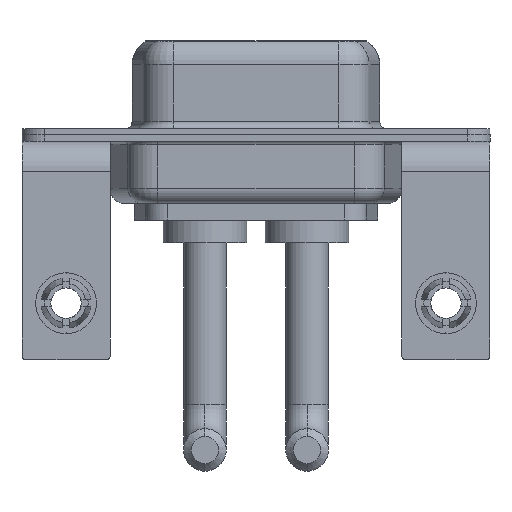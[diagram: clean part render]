
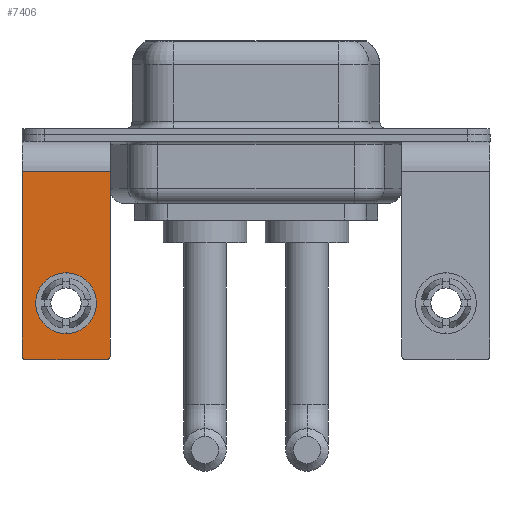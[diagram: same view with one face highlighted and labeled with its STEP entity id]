
A CAD part, front view. The second image highlights one B-rep face of the part: STEP entity #7406.
In plain terms, the highlighted planar face has unit normal (0, -1, 0).
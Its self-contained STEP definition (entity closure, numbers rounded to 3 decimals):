
#21 = VECTOR ( 'NONE', #13618, 1000. ) ;
#364 = CARTESIAN_POINT ( 'NONE',  ( 0., -6.25, -11.07 ) ) ;
#585 = DIRECTION ( 'NONE',  ( 0., -1., 0. ) ) ;
#714 = DIRECTION ( 'NONE',  ( -1., 0., 0. ) ) ;
#743 = ORIENTED_EDGE ( 'NONE', *, *, #3849, .F. ) ;
#789 = DIRECTION ( 'NONE',  ( 0., 1., 0. ) ) ;
#862 = CARTESIAN_POINT ( 'NONE',  ( 0., -6.25, -11.07 ) ) ;
#1031 = PLANE ( 'NONE',  #11080 ) ;
#1300 = EDGE_LOOP ( 'NONE', ( #14011, #5399, #4570, #6254, #743, #12865 ) ) ;
#1402 = VERTEX_POINT ( 'NONE', #13910 ) ;
#1481 = CARTESIAN_POINT ( 'NONE',  ( 0., -6.25, -13.07 ) ) ;
#1553 = CIRCLE ( 'NONE', #11958, 0.25 ) ;
#1920 = ORIENTED_EDGE ( 'NONE', *, *, #5499, .T. ) ;
#2193 = CARTESIAN_POINT ( 'NONE',  ( 2.9, -6.25, -14.55 ) ) ;
#2292 = VERTEX_POINT ( 'NONE', #8793 ) ;
#2634 = EDGE_CURVE ( 'NONE', #6233, #2292, #1553, .T. ) ;
#3094 = AXIS2_PLACEMENT_3D ( 'NONE', #862, #789, #9762 ) ;
#3145 = LINE ( 'NONE', #5505, #4520 ) ;
#3213 = CARTESIAN_POINT ( 'NONE',  ( 0., -6.25, -9.07 ) ) ;
#3627 = DIRECTION ( 'NONE',  ( 0., 0., -1. ) ) ;
#3849 = EDGE_CURVE ( 'NONE', #1402, #5705, #4943, .T. ) ;
#4283 = CARTESIAN_POINT ( 'NONE',  ( 2.65, -6.25, -14.8 ) ) ;
#4520 = VECTOR ( 'NONE', #714, 1000. ) ;
#4570 = ORIENTED_EDGE ( 'NONE', *, *, #10517, .F. ) ;
#4727 = DIRECTION ( 'NONE',  ( 0., 0., 1. ) ) ;
#4874 = LINE ( 'NONE', #5689, #21 ) ;
#4943 = LINE ( 'NONE', #10308, #11025 ) ;
#5083 = DIRECTION ( 'NONE',  ( 0., 0., 1. ) ) ;
#5118 = VERTEX_POINT ( 'NONE', #1481 ) ;
#5286 = VERTEX_POINT ( 'NONE', #4283 ) ;
#5399 = ORIENTED_EDGE ( 'NONE', *, *, #2634, .T. ) ;
#5499 = EDGE_CURVE ( 'NONE', #10412, #5118, #9878, .T. ) ;
#5505 = CARTESIAN_POINT ( 'NONE',  ( 2.9, -6.25, -2.4 ) ) ;
#5668 = DIRECTION ( 'NONE',  ( 0., 0., 1. ) ) ;
#5689 = CARTESIAN_POINT ( 'NONE',  ( -2.9, -6.25, -2.4 ) ) ;
#5705 = VERTEX_POINT ( 'NONE', #2193 ) ;
#5760 = EDGE_LOOP ( 'NONE', ( #13253, #1920 ) ) ;
#6233 = VERTEX_POINT ( 'NONE', #13499 ) ;
#6254 = ORIENTED_EDGE ( 'NONE', *, *, #7365, .T. ) ;
#6545 = FACE_OUTER_BOUND ( 'NONE', #1300, .T. ) ;
#7044 = LINE ( 'NONE', #8225, #11607 ) ;
#7159 = EDGE_CURVE ( 'NONE', #7710, #6233, #4874, .T. ) ;
#7298 = AXIS2_PLACEMENT_3D ( 'NONE', #11762, #585, #5083 ) ;
#7365 = EDGE_CURVE ( 'NONE', #5286, #5705, #8018, .T. ) ;
#7406 = ADVANCED_FACE ( 'NONE', ( #8607, #6545 ), #1031, .F. ) ;
#7583 = DIRECTION ( 'NONE',  ( 0., 0., 1. ) ) ;
#7710 = VERTEX_POINT ( 'NONE', #10290 ) ;
#7875 = DIRECTION ( 'NONE',  ( 0., -1., 0. ) ) ;
#7945 = EDGE_CURVE ( 'NONE', #1402, #7710, #3145, .T. ) ;
#8018 = CIRCLE ( 'NONE', #7298, 0.25 ) ;
#8026 = EDGE_CURVE ( 'NONE', #5118, #10412, #9907, .T. ) ;
#8225 = CARTESIAN_POINT ( 'NONE',  ( 2.9, -6.25, -14.8 ) ) ;
#8607 = FACE_BOUND ( 'NONE', #5760, .T. ) ;
#8793 = CARTESIAN_POINT ( 'NONE',  ( -2.65, -6.25, -14.8 ) ) ;
#9183 = AXIS2_PLACEMENT_3D ( 'NONE', #364, #12859, #4727 ) ;
#9762 = DIRECTION ( 'NONE',  ( 0., 0., 1. ) ) ;
#9878 = CIRCLE ( 'NONE', #9183, 2. ) ;
#9907 = CIRCLE ( 'NONE', #3094, 2. ) ;
#10003 = DIRECTION ( 'NONE',  ( 0., 1., 0. ) ) ;
#10290 = CARTESIAN_POINT ( 'NONE',  ( -2.9, -6.25, -2.4 ) ) ;
#10308 = CARTESIAN_POINT ( 'NONE',  ( 2.9, -6.25, -2.4 ) ) ;
#10412 = VERTEX_POINT ( 'NONE', #3213 ) ;
#10517 = EDGE_CURVE ( 'NONE', #5286, #2292, #7044, .T. ) ;
#10877 = CARTESIAN_POINT ( 'NONE',  ( 2.9, -6.25, -2.4 ) ) ;
#11025 = VECTOR ( 'NONE', #3627, 1000. ) ;
#11080 = AXIS2_PLACEMENT_3D ( 'NONE', #10877, #10003, #7583 ) ;
#11311 = DIRECTION ( 'NONE',  ( -1., 0., 0. ) ) ;
#11607 = VECTOR ( 'NONE', #11311, 1000. ) ;
#11762 = CARTESIAN_POINT ( 'NONE',  ( 2.65, -6.25, -14.55 ) ) ;
#11958 = AXIS2_PLACEMENT_3D ( 'NONE', #13313, #7875, #5668 ) ;
#12859 = DIRECTION ( 'NONE',  ( 0., 1., 0. ) ) ;
#12865 = ORIENTED_EDGE ( 'NONE', *, *, #7945, .T. ) ;
#13253 = ORIENTED_EDGE ( 'NONE', *, *, #8026, .T. ) ;
#13313 = CARTESIAN_POINT ( 'NONE',  ( -2.65, -6.25, -14.55 ) ) ;
#13499 = CARTESIAN_POINT ( 'NONE',  ( -2.9, -6.25, -14.55 ) ) ;
#13618 = DIRECTION ( 'NONE',  ( 0., 0., -1. ) ) ;
#13910 = CARTESIAN_POINT ( 'NONE',  ( 2.9, -6.25, -2.4 ) ) ;
#14011 = ORIENTED_EDGE ( 'NONE', *, *, #7159, .T. ) ;
